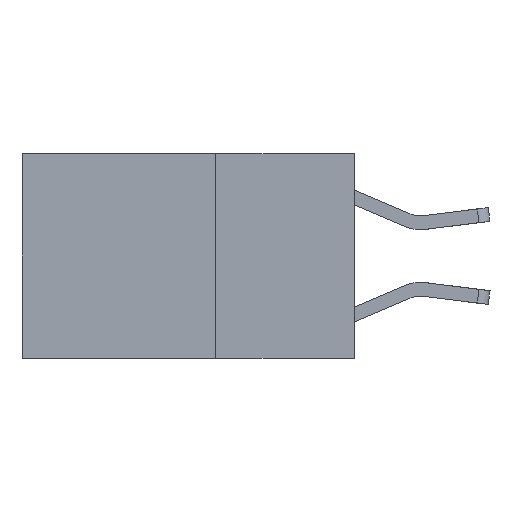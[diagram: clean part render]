
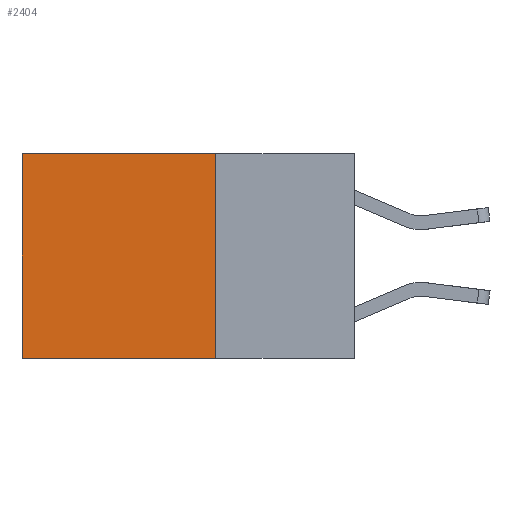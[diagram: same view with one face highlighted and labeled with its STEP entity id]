
A CAD part, left-side view. The second image highlights one B-rep face of the part: STEP entity #2404.
In plain terms, the highlighted planar face has unit normal (-1, 0, 0).
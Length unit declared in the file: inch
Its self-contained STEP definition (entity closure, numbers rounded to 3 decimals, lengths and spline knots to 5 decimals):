
#59 = DIRECTION ( 'NONE',  ( 1., 0., 0. ) ) ;
#657 = VERTEX_POINT ( 'NONE', #4177 ) ;
#730 = DIRECTION ( 'NONE',  ( 0., 0., -1. ) ) ;
#943 = CARTESIAN_POINT ( 'NONE',  ( 0.2625, 0.6, 0. ) ) ;
#1318 = LINE ( 'NONE', #7965, #10381 ) ;
#1671 = LINE ( 'NONE', #8700, #2800 ) ;
#1823 = CARTESIAN_POINT ( 'NONE',  ( 0.2625, 0.25, 0. ) ) ;
#1860 = ORIENTED_EDGE ( 'NONE', *, *, #3302, .F. ) ;
#2263 = AXIS2_PLACEMENT_3D ( 'NONE', #1823, #59, #10697 ) ;
#2404 = ADVANCED_FACE ( 'NONE', ( #4176 ), #8037, .F. ) ;
#2800 = VECTOR ( 'NONE', #5114, 39.37008 ) ;
#3302 = EDGE_CURVE ( 'NONE', #11232, #657, #6466, .T. ) ;
#3625 = VECTOR ( 'NONE', #11362, 39.37008 ) ;
#3664 = EDGE_CURVE ( 'NONE', #8523, #657, #8545, .T. ) ;
#3775 = EDGE_CURVE ( 'NONE', #6131, #11232, #1318, .T. ) ;
#4176 = FACE_OUTER_BOUND ( 'NONE', #4314, .T. ) ;
#4177 = CARTESIAN_POINT ( 'NONE',  ( 0.2625, 0.6, -0.37 ) ) ;
#4314 = EDGE_LOOP ( 'NONE', ( #4755, #1860, #7060, #6428 ) ) ;
#4755 = ORIENTED_EDGE ( 'NONE', *, *, #3664, .T. ) ;
#5114 = DIRECTION ( 'NONE',  ( 0., 1., 0. ) ) ;
#5592 = VECTOR ( 'NONE', #730, 39.37008 ) ;
#6131 = VERTEX_POINT ( 'NONE', #10610 ) ;
#6428 = ORIENTED_EDGE ( 'NONE', *, *, #11318, .T. ) ;
#6466 = LINE ( 'NONE', #8604, #3625 ) ;
#7060 = ORIENTED_EDGE ( 'NONE', *, *, #3775, .F. ) ;
#7965 = CARTESIAN_POINT ( 'NONE',  ( 0.2625, 0.25, 0. ) ) ;
#8037 = PLANE ( 'NONE',  #2263 ) ;
#8523 = VERTEX_POINT ( 'NONE', #943 ) ;
#8545 = LINE ( 'NONE', #8956, #5592 ) ;
#8604 = CARTESIAN_POINT ( 'NONE',  ( 0.2625, 0.25, -0.37 ) ) ;
#8700 = CARTESIAN_POINT ( 'NONE',  ( 0.2625, 0.25, 0. ) ) ;
#8956 = CARTESIAN_POINT ( 'NONE',  ( 0.2625, 0.6, 0. ) ) ;
#10381 = VECTOR ( 'NONE', #10693, 39.37008 ) ;
#10520 = CARTESIAN_POINT ( 'NONE',  ( 0.2625, 0.25, -0.37 ) ) ;
#10610 = CARTESIAN_POINT ( 'NONE',  ( 0.2625, 0.25, 0. ) ) ;
#10693 = DIRECTION ( 'NONE',  ( 0., 0., -1. ) ) ;
#10697 = DIRECTION ( 'NONE',  ( 0., 0., -1. ) ) ;
#11232 = VERTEX_POINT ( 'NONE', #10520 ) ;
#11318 = EDGE_CURVE ( 'NONE', #6131, #8523, #1671, .T. ) ;
#11362 = DIRECTION ( 'NONE',  ( 0., 1., 0. ) ) ;
